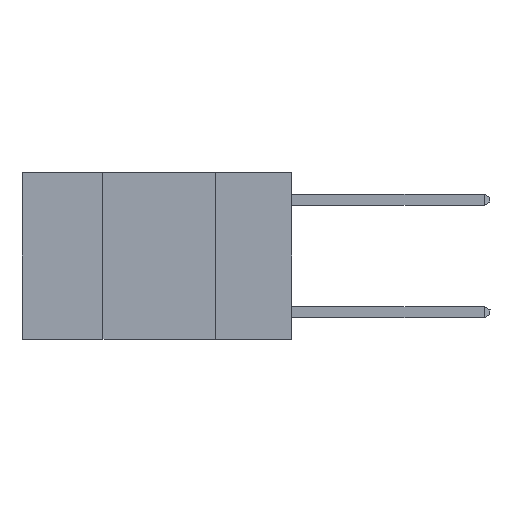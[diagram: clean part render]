
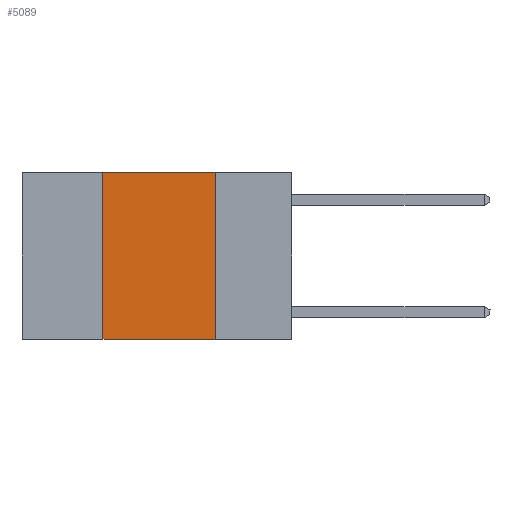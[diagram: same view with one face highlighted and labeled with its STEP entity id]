
A CAD part, left-side view. The second image highlights one B-rep face of the part: STEP entity #5089.
In plain terms, the highlighted planar face has unit normal (-1, 0, 0).
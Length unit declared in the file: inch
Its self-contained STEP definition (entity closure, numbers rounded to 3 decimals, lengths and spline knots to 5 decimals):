
#212 = EDGE_LOOP ( 'NONE', ( #623, #9230, #9030, #5506 ) ) ;
#623 = ORIENTED_EDGE ( 'NONE', *, *, #2577, .F. ) ;
#783 = LINE ( 'NONE', #3509, #6738 ) ;
#1800 = VECTOR ( 'NONE', #9798, 39.37008 ) ;
#2305 = VERTEX_POINT ( 'NONE', #7858 ) ;
#2394 = CARTESIAN_POINT ( 'NONE',  ( 0., 0.42, 0. ) ) ;
#2577 = EDGE_CURVE ( 'NONE', #3251, #2305, #6870, .T. ) ;
#2838 = VECTOR ( 'NONE', #2890, 39.37008 ) ;
#2890 = DIRECTION ( 'NONE',  ( 0., -1., 0. ) ) ;
#2968 = CARTESIAN_POINT ( 'NONE',  ( 0., 0.42, -0.37 ) ) ;
#3077 = CARTESIAN_POINT ( 'NONE',  ( 0., 0.6, 0. ) ) ;
#3251 = VERTEX_POINT ( 'NONE', #9619 ) ;
#3320 = EDGE_CURVE ( 'NONE', #4145, #4056, #783, .T. ) ;
#3356 = PLANE ( 'NONE',  #4770 ) ;
#3509 = CARTESIAN_POINT ( 'NONE',  ( 0., 0.42, 0. ) ) ;
#3785 = LINE ( 'NONE', #3077, #1800 ) ;
#3800 = CARTESIAN_POINT ( 'NONE',  ( 0., 0.17, 0. ) ) ;
#4056 = VERTEX_POINT ( 'NONE', #2394 ) ;
#4145 = VERTEX_POINT ( 'NONE', #2968 ) ;
#4770 = AXIS2_PLACEMENT_3D ( 'NONE', #5617, #9352, #4826 ) ;
#4801 = LINE ( 'NONE', #6762, #2838 ) ;
#4826 = DIRECTION ( 'NONE',  ( 0., 0., -1. ) ) ;
#5089 = ADVANCED_FACE ( 'NONE', ( #5782 ), #3356, .F. ) ;
#5506 = ORIENTED_EDGE ( 'NONE', *, *, #8581, .T. ) ;
#5617 = CARTESIAN_POINT ( 'NONE',  ( 0., 0.6, 0. ) ) ;
#5782 = FACE_OUTER_BOUND ( 'NONE', #212, .T. ) ;
#6625 = VECTOR ( 'NONE', #9211, 39.37008 ) ;
#6738 = VECTOR ( 'NONE', #9756, 39.37008 ) ;
#6762 = CARTESIAN_POINT ( 'NONE',  ( 0., 0.6, -0.37 ) ) ;
#6870 = LINE ( 'NONE', #3800, #6625 ) ;
#7858 = CARTESIAN_POINT ( 'NONE',  ( 0., 0.17, -0.37 ) ) ;
#7936 = EDGE_CURVE ( 'NONE', #4056, #3251, #3785, .T. ) ;
#8581 = EDGE_CURVE ( 'NONE', #4145, #2305, #4801, .T. ) ;
#9030 = ORIENTED_EDGE ( 'NONE', *, *, #3320, .F. ) ;
#9211 = DIRECTION ( 'NONE',  ( 0., 0., -1. ) ) ;
#9230 = ORIENTED_EDGE ( 'NONE', *, *, #7936, .F. ) ;
#9352 = DIRECTION ( 'NONE',  ( 1., 0., 0. ) ) ;
#9619 = CARTESIAN_POINT ( 'NONE',  ( 0., 0.17, 0. ) ) ;
#9756 = DIRECTION ( 'NONE',  ( 0., 0., 1. ) ) ;
#9798 = DIRECTION ( 'NONE',  ( 0., -1., 0. ) ) ;
